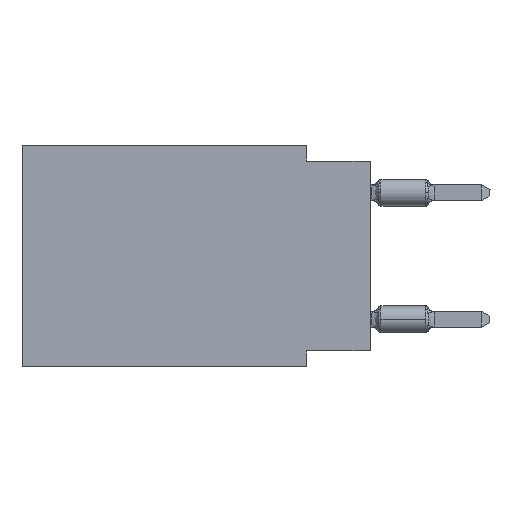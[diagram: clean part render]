
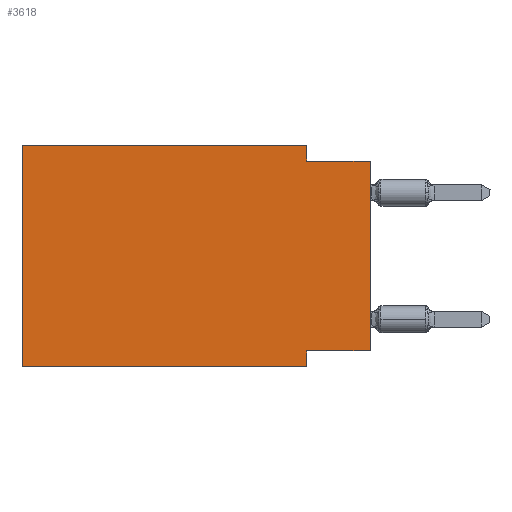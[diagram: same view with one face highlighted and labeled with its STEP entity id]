
A CAD part, left-side view. The second image highlights one B-rep face of the part: STEP entity #3618.
In plain terms, the highlighted planar face has unit normal (-1, 0, 0).
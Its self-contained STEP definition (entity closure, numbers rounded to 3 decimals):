
#20 = LINE ( 'NONE', #13968, #4643 ) ;
#1363 = VECTOR ( 'NONE', #3842, 1000. ) ;
#2913 = CARTESIAN_POINT ( 'NONE',  ( 0., 0., -8.255 ) ) ;
#2989 = EDGE_LOOP ( 'NONE', ( #15903, #31280, #9284, #9555, #14176, #9207, #19792, #44852 ) ) ;
#3401 = AXIS2_PLACEMENT_3D ( 'NONE', #27363, #38335, #20754 ) ;
#3618 = ADVANCED_FACE ( 'NONE', ( #28655 ), #6579, .F. ) ;
#3842 = DIRECTION ( 'NONE',  ( 0., 0., -1. ) ) ;
#4305 = LINE ( 'NONE', #25514, #1363 ) ;
#4643 = VECTOR ( 'NONE', #27875, 1000. ) ;
#4667 = VERTEX_POINT ( 'NONE', #40421 ) ;
#4689 = CARTESIAN_POINT ( 'NONE',  ( 0., 13.97, 0. ) ) ;
#5794 = VERTEX_POINT ( 'NONE', #29322 ) ;
#5984 = VERTEX_POINT ( 'NONE', #9688 ) ;
#6579 = PLANE ( 'NONE',  #3401 ) ;
#8386 = EDGE_CURVE ( 'NONE', #5794, #14960, #4305, .T. ) ;
#9207 = ORIENTED_EDGE ( 'NONE', *, *, #32850, .T. ) ;
#9284 = ORIENTED_EDGE ( 'NONE', *, *, #8386, .F. ) ;
#9555 = ORIENTED_EDGE ( 'NONE', *, *, #37660, .F. ) ;
#9688 = CARTESIAN_POINT ( 'NONE',  ( 0., 0., -8.255 ) ) ;
#11400 = EDGE_CURVE ( 'NONE', #5984, #4667, #45041, .T. ) ;
#12515 = DIRECTION ( 'NONE',  ( 0., 1., 0. ) ) ;
#12637 = LINE ( 'NONE', #19043, #39700 ) ;
#13968 = CARTESIAN_POINT ( 'NONE',  ( 0., 2.54, -8.89 ) ) ;
#14176 = ORIENTED_EDGE ( 'NONE', *, *, #43507, .F. ) ;
#14960 = VERTEX_POINT ( 'NONE', #29133 ) ;
#15523 = VERTEX_POINT ( 'NONE', #32168 ) ;
#15903 = ORIENTED_EDGE ( 'NONE', *, *, #11400, .T. ) ;
#17124 = LINE ( 'NONE', #4689, #44849 ) ;
#17986 = CARTESIAN_POINT ( 'NONE',  ( 0., 13.97, 0. ) ) ;
#19043 = CARTESIAN_POINT ( 'NONE',  ( 0., 0., -0.635 ) ) ;
#19240 = VECTOR ( 'NONE', #35718, 1000. ) ;
#19792 = ORIENTED_EDGE ( 'NONE', *, *, #42733, .F. ) ;
#20641 = EDGE_CURVE ( 'NONE', #14960, #4667, #12637, .T. ) ;
#20754 = DIRECTION ( 'NONE',  ( 0., 0., -1. ) ) ;
#21462 = VERTEX_POINT ( 'NONE', #30085 ) ;
#21632 = DIRECTION ( 'NONE',  ( 0., 0., 1. ) ) ;
#22470 = VECTOR ( 'NONE', #12515, 1000. ) ;
#24006 = CARTESIAN_POINT ( 'NONE',  ( 0., 0., 0. ) ) ;
#24597 = LINE ( 'NONE', #17986, #34596 ) ;
#25055 = CARTESIAN_POINT ( 'NONE',  ( 0., 2.54, -8.89 ) ) ;
#25514 = CARTESIAN_POINT ( 'NONE',  ( 0., 2.54, 0. ) ) ;
#27363 = CARTESIAN_POINT ( 'NONE',  ( 0., 13.97, 0. ) ) ;
#27875 = DIRECTION ( 'NONE',  ( 0., 0., -1. ) ) ;
#28613 = VERTEX_POINT ( 'NONE', #44899 ) ;
#28655 = FACE_OUTER_BOUND ( 'NONE', #2989, .T. ) ;
#29133 = CARTESIAN_POINT ( 'NONE',  ( 0., 2.54, -0.635 ) ) ;
#29285 = CARTESIAN_POINT ( 'NONE',  ( 0., 13.97, -8.89 ) ) ;
#29322 = CARTESIAN_POINT ( 'NONE',  ( 0., 2.54, 0. ) ) ;
#29502 = VERTEX_POINT ( 'NONE', #25055 ) ;
#30085 = CARTESIAN_POINT ( 'NONE',  ( 0., 13.97, 0. ) ) ;
#30196 = DIRECTION ( 'NONE',  ( 0., -1., 0. ) ) ;
#30871 = EDGE_CURVE ( 'NONE', #5984, #28613, #36954, .T. ) ;
#31280 = ORIENTED_EDGE ( 'NONE', *, *, #20641, .F. ) ;
#32168 = CARTESIAN_POINT ( 'NONE',  ( 0., 13.97, -8.89 ) ) ;
#32850 = EDGE_CURVE ( 'NONE', #15523, #29502, #42806, .T. ) ;
#34596 = VECTOR ( 'NONE', #21632, 1000. ) ;
#34960 = DIRECTION ( 'NONE',  ( 0., 0., 1. ) ) ;
#35718 = DIRECTION ( 'NONE',  ( 0., -1., 0. ) ) ;
#36954 = LINE ( 'NONE', #2913, #22470 ) ;
#37660 = EDGE_CURVE ( 'NONE', #21462, #5794, #17124, .T. ) ;
#38335 = DIRECTION ( 'NONE',  ( 1., 0., 0. ) ) ;
#39191 = DIRECTION ( 'NONE',  ( 0., -1., 0. ) ) ;
#39700 = VECTOR ( 'NONE', #30196, 1000. ) ;
#40421 = CARTESIAN_POINT ( 'NONE',  ( 0., 0., -0.635 ) ) ;
#41961 = VECTOR ( 'NONE', #34960, 1000. ) ;
#42733 = EDGE_CURVE ( 'NONE', #28613, #29502, #20, .T. ) ;
#42806 = LINE ( 'NONE', #29285, #19240 ) ;
#43507 = EDGE_CURVE ( 'NONE', #15523, #21462, #24597, .T. ) ;
#44849 = VECTOR ( 'NONE', #39191, 1000. ) ;
#44852 = ORIENTED_EDGE ( 'NONE', *, *, #30871, .F. ) ;
#44899 = CARTESIAN_POINT ( 'NONE',  ( 0., 2.54, -8.255 ) ) ;
#45041 = LINE ( 'NONE', #24006, #41961 ) ;
